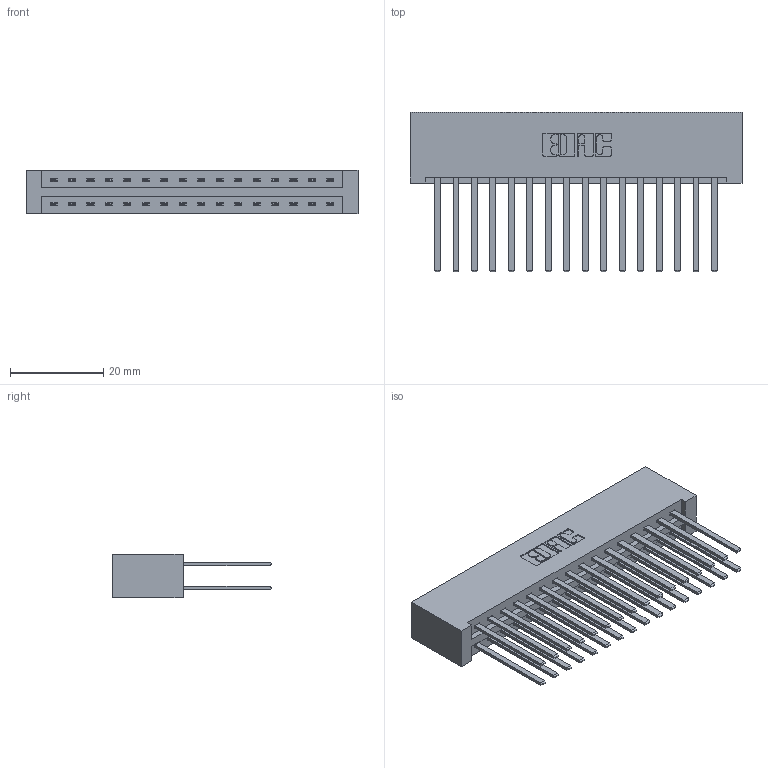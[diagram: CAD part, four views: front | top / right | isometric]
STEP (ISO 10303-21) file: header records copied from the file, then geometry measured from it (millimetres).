
FILE_DESCRIPTION (( 'STEP AP203' ), '1' );
FILE_NAME ('387-032-544-201.STEP', '2019-10-17T16:06:16', ( '' ), ( '' ), 'SwSTEP 2.0', 'SolidWorks 2016', '' );
FILE_SCHEMA (( 'CONFIG_CONTROL_DESIGN' ));
Length unit declared in the file: inch
Products named in the file (3): 387-032-544-201; 337 Part_No Mounting Lugs; 345-292-001_345-293-144
Assembly tree (33 placements, depth 2):
  387-032-544-201
    337 Part_No Mounting Lugs
    345-292-001_345-293-144  x32
Bounding box: 71.27 x 34.3 x 9.4 mm (x, y, z)
Volume: 8374.5 mm3; surface area: 10736.3 mm2
Topology: 33 solids, 33 shells, 1642 faces, 4863 edges, 3198 vertices
Faces by surface type: plane 1154, cylinder 488
Entity records: 15307 total; most frequent: CARTESIAN_POINT 2598, ORIENTED_EDGE 2534, DIRECTION 2247, EDGE_CURVE 1267, LINE 1151, VECTOR 1151, VERTEX_POINT 842, AXIS2_PLACEMENT_3D 548
